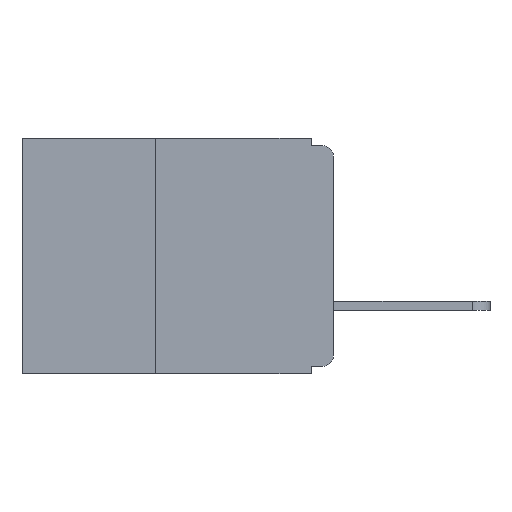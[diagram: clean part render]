
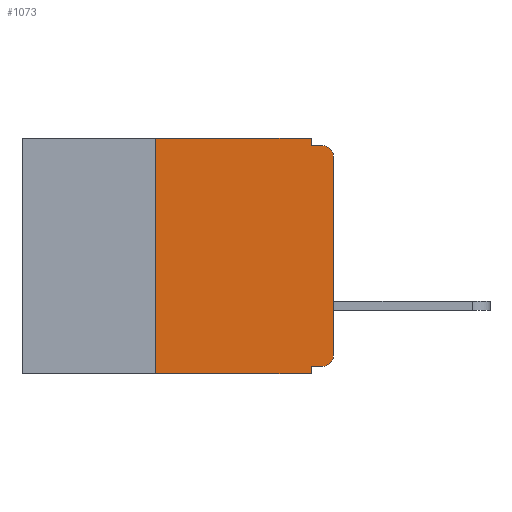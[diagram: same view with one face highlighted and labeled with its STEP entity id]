
A CAD part, left-side view. The second image highlights one B-rep face of the part: STEP entity #1073.
In plain terms, the highlighted planar face has unit normal (-1, 0, 0).
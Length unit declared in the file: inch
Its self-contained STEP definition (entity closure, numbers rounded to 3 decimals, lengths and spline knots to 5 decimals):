
#289 = CIRCLE ( 'NONE', #10989, 0.015 ) ;
#305 = DIRECTION ( 'NONE',  ( -1., 0., 0. ) ) ;
#490 = ORIENTED_EDGE ( 'NONE', *, *, #30806, .T. ) ;
#1073 = ADVANCED_FACE ( 'NONE', ( #2744 ), #9925, .F. ) ;
#1423 = VECTOR ( 'NONE', #12100, 39.37008 ) ;
#2744 = FACE_OUTER_BOUND ( 'NONE', #31558, .T. ) ;
#3055 = CARTESIAN_POINT ( 'NONE',  ( 0., 0.031, -0.32 ) ) ;
#3657 = DIRECTION ( 'NONE',  ( 0., 0., -1. ) ) ;
#3702 = ORIENTED_EDGE ( 'NONE', *, *, #14952, .F. ) ;
#4053 = EDGE_CURVE ( 'NONE', #17672, #20641, #11116, .T. ) ;
#4082 = VECTOR ( 'NONE', #28731, 39.37008 ) ;
#4195 = VECTOR ( 'NONE', #20887, 39.37008 ) ;
#4242 = EDGE_CURVE ( 'NONE', #28907, #26839, #22414, .T. ) ;
#5185 = VERTEX_POINT ( 'NONE', #19839 ) ;
#5384 = LINE ( 'NONE', #29740, #32290 ) ;
#5825 = EDGE_CURVE ( 'NONE', #5185, #32818, #289, .T. ) ;
#6237 = CARTESIAN_POINT ( 'NONE',  ( 0., 0.031, -0.33 ) ) ;
#6278 = EDGE_CURVE ( 'NONE', #7061, #17672, #6399, .T. ) ;
#6399 = LINE ( 'NONE', #9197, #33282 ) ;
#6480 = CIRCLE ( 'NONE', #15930, 0.015 ) ;
#6907 = EDGE_CURVE ( 'NONE', #22417, #11855, #12871, .T. ) ;
#7045 = CARTESIAN_POINT ( 'NONE',  ( 0., 0., -0.025 ) ) ;
#7061 = VERTEX_POINT ( 'NONE', #25631 ) ;
#7394 = CARTESIAN_POINT ( 'NONE',  ( 0., 0.015, -0.305 ) ) ;
#7437 = ORIENTED_EDGE ( 'NONE', *, *, #4242, .F. ) ;
#7852 = CARTESIAN_POINT ( 'NONE',  ( 0., 0.25, 0. ) ) ;
#9197 = CARTESIAN_POINT ( 'NONE',  ( 0., 0.25, -0.33 ) ) ;
#9308 = DIRECTION ( 'NONE',  ( 0., 0., 1. ) ) ;
#9337 = DIRECTION ( 'NONE',  ( 1., 0., 0. ) ) ;
#9446 = DIRECTION ( 'NONE',  ( 0., 0., -1. ) ) ;
#9925 = PLANE ( 'NONE',  #20252 ) ;
#10010 = DIRECTION ( 'NONE',  ( 0., 0., -1. ) ) ;
#10098 = ORIENTED_EDGE ( 'NONE', *, *, #4053, .F. ) ;
#10979 = EDGE_CURVE ( 'NONE', #7061, #11855, #14604, .T. ) ;
#10989 = AXIS2_PLACEMENT_3D ( 'NONE', #7394, #25596, #10010 ) ;
#11026 = CARTESIAN_POINT ( 'NONE',  ( 0., 0., -0.32 ) ) ;
#11116 = LINE ( 'NONE', #20997, #4195 ) ;
#11855 = VERTEX_POINT ( 'NONE', #6237 ) ;
#11928 = ORIENTED_EDGE ( 'NONE', *, *, #17165, .T. ) ;
#12100 = DIRECTION ( 'NONE',  ( 0., 0., -1. ) ) ;
#12871 = LINE ( 'NONE', #27683, #1423 ) ;
#13649 = EDGE_CURVE ( 'NONE', #5185, #22417, #28241, .T. ) ;
#13721 = CARTESIAN_POINT ( 'NONE',  ( 0., 0.031, 0. ) ) ;
#14604 = LINE ( 'NONE', #18347, #27610 ) ;
#14952 = EDGE_CURVE ( 'NONE', #20641, #28907, #5384, .T. ) ;
#15930 = AXIS2_PLACEMENT_3D ( 'NONE', #15940, #305, #18553 ) ;
#15940 = CARTESIAN_POINT ( 'NONE',  ( 0., 0.015, -0.025 ) ) ;
#17165 = EDGE_CURVE ( 'NONE', #32818, #24553, #17906, .T. ) ;
#17672 = VERTEX_POINT ( 'NONE', #7852 ) ;
#17733 = DIRECTION ( 'NONE',  ( 0., -1., 0. ) ) ;
#17868 = CARTESIAN_POINT ( 'NONE',  ( 0., 0., -0.01 ) ) ;
#17906 = LINE ( 'NONE', #26101, #4082 ) ;
#18347 = CARTESIAN_POINT ( 'NONE',  ( 0., 0.437, -0.33 ) ) ;
#18553 = DIRECTION ( 'NONE',  ( 0., 0., -1. ) ) ;
#18693 = ORIENTED_EDGE ( 'NONE', *, *, #5825, .T. ) ;
#19008 = CARTESIAN_POINT ( 'NONE',  ( 0., 0., -0.305 ) ) ;
#19839 = CARTESIAN_POINT ( 'NONE',  ( 0., 0.015, -0.32 ) ) ;
#20227 = CARTESIAN_POINT ( 'NONE',  ( 0., 0.437, 0. ) ) ;
#20252 = AXIS2_PLACEMENT_3D ( 'NONE', #20227, #9337, #9446 ) ;
#20468 = CARTESIAN_POINT ( 'NONE',  ( 0., 0.031, -0.01 ) ) ;
#20641 = VERTEX_POINT ( 'NONE', #13721 ) ;
#20887 = DIRECTION ( 'NONE',  ( 0., -1., 0. ) ) ;
#20944 = DIRECTION ( 'NONE',  ( 0., -1., 0. ) ) ;
#20997 = CARTESIAN_POINT ( 'NONE',  ( 0., 0.437, 0. ) ) ;
#22414 = LINE ( 'NONE', #17868, #28537 ) ;
#22417 = VERTEX_POINT ( 'NONE', #3055 ) ;
#24553 = VERTEX_POINT ( 'NONE', #7045 ) ;
#25596 = DIRECTION ( 'NONE',  ( -1., 0., 0. ) ) ;
#25631 = CARTESIAN_POINT ( 'NONE',  ( 0., 0.25, -0.33 ) ) ;
#26101 = CARTESIAN_POINT ( 'NONE',  ( 0., 0., 0. ) ) ;
#26235 = ORIENTED_EDGE ( 'NONE', *, *, #10979, .T. ) ;
#26839 = VERTEX_POINT ( 'NONE', #32656 ) ;
#27433 = VECTOR ( 'NONE', #29249, 39.37008 ) ;
#27610 = VECTOR ( 'NONE', #20944, 39.37008 ) ;
#27683 = CARTESIAN_POINT ( 'NONE',  ( 0., 0.031, -0.33 ) ) ;
#28241 = LINE ( 'NONE', #11026, #27433 ) ;
#28537 = VECTOR ( 'NONE', #17733, 39.37008 ) ;
#28730 = ORIENTED_EDGE ( 'NONE', *, *, #6907, .F. ) ;
#28731 = DIRECTION ( 'NONE',  ( 0., 0., 1. ) ) ;
#28907 = VERTEX_POINT ( 'NONE', #20468 ) ;
#29249 = DIRECTION ( 'NONE',  ( 0., 1., 0. ) ) ;
#29740 = CARTESIAN_POINT ( 'NONE',  ( 0., 0.031, 0. ) ) ;
#30806 = EDGE_CURVE ( 'NONE', #24553, #26839, #6480, .T. ) ;
#30916 = ORIENTED_EDGE ( 'NONE', *, *, #13649, .F. ) ;
#31558 = EDGE_LOOP ( 'NONE', ( #11928, #490, #7437, #3702, #10098, #33814, #26235, #28730, #30916, #18693 ) ) ;
#32290 = VECTOR ( 'NONE', #3657, 39.37008 ) ;
#32656 = CARTESIAN_POINT ( 'NONE',  ( 0., 0.015, -0.01 ) ) ;
#32818 = VERTEX_POINT ( 'NONE', #19008 ) ;
#33282 = VECTOR ( 'NONE', #9308, 39.37008 ) ;
#33814 = ORIENTED_EDGE ( 'NONE', *, *, #6278, .F. ) ;
